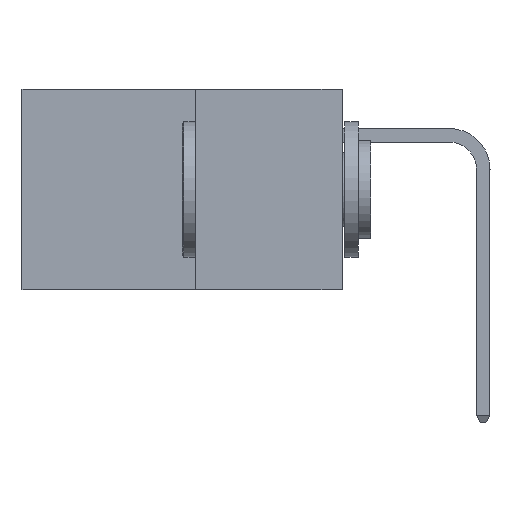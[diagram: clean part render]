
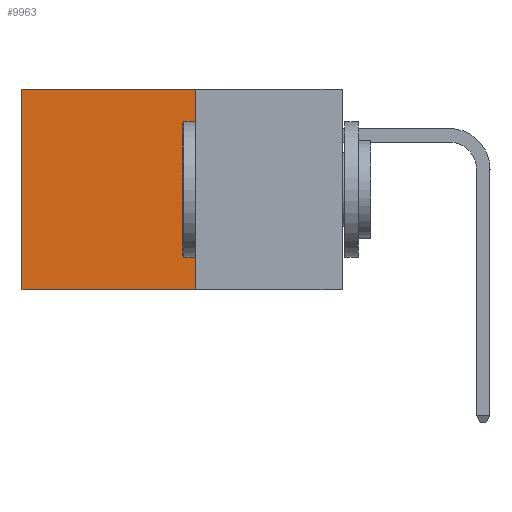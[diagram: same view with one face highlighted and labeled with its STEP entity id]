
A CAD part, left-side view. The second image highlights one B-rep face of the part: STEP entity #9963.
In plain terms, the highlighted planar face has unit normal (-1, 0, 0).
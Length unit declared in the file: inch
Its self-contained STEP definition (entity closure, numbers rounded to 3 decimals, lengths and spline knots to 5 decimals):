
#139 = DIRECTION ( 'NONE',  ( 0., 0., -1. ) ) ;
#162 = DIRECTION ( 'NONE',  ( 1., 0., 0. ) ) ;
#205 = CARTESIAN_POINT ( 'NONE',  ( 0.277, 0.27, -0.37 ) ) ;
#328 = CARTESIAN_POINT ( 'NONE',  ( 0.277, 0.27, -0.37 ) ) ;
#773 = PLANE ( 'NONE',  #18430 ) ;
#1620 = DIRECTION ( 'NONE',  ( 0., 1., 0. ) ) ;
#2046 = DIRECTION ( 'NONE',  ( 0., 0., -1. ) ) ;
#2365 = FACE_OUTER_BOUND ( 'NONE', #10256, .T. ) ;
#3644 = ORIENTED_EDGE ( 'NONE', *, *, #20527, .F. ) ;
#3859 = LINE ( 'NONE', #21439, #12169 ) ;
#5663 = EDGE_CURVE ( 'NONE', #18821, #10650, #12101, .T. ) ;
#6355 = DIRECTION ( 'NONE',  ( 0., 1., 0. ) ) ;
#7177 = VECTOR ( 'NONE', #15271, 39.37008 ) ;
#7465 = VERTEX_POINT ( 'NONE', #9952 ) ;
#9685 = VECTOR ( 'NONE', #2046, 39.37008 ) ;
#9881 = ORIENTED_EDGE ( 'NONE', *, *, #5663, .T. ) ;
#9952 = CARTESIAN_POINT ( 'NONE',  ( 0.277, 0.27, -0.37 ) ) ;
#9963 = ADVANCED_FACE ( 'NONE', ( #2365 ), #773, .F. ) ;
#10256 = EDGE_LOOP ( 'NONE', ( #9881, #3644, #15659, #20022 ) ) ;
#10650 = VERTEX_POINT ( 'NONE', #17677 ) ;
#11671 = EDGE_CURVE ( 'NONE', #20823, #7465, #14165, .T. ) ;
#11975 = VECTOR ( 'NONE', #6355, 39.37008 ) ;
#12101 = LINE ( 'NONE', #15163, #7177 ) ;
#12169 = VECTOR ( 'NONE', #1620, 39.37008 ) ;
#12953 = CARTESIAN_POINT ( 'NONE',  ( 0.277, 0.27, 0. ) ) ;
#14165 = LINE ( 'NONE', #328, #9685 ) ;
#15163 = CARTESIAN_POINT ( 'NONE',  ( 0.277, 0.59, -0.37 ) ) ;
#15271 = DIRECTION ( 'NONE',  ( 0., 0., -1. ) ) ;
#15561 = CARTESIAN_POINT ( 'NONE',  ( 0.277, 0.27, 0. ) ) ;
#15659 = ORIENTED_EDGE ( 'NONE', *, *, #11671, .F. ) ;
#16424 = LINE ( 'NONE', #12953, #11975 ) ;
#17677 = CARTESIAN_POINT ( 'NONE',  ( 0.277, 0.59, -0.37 ) ) ;
#18430 = AXIS2_PLACEMENT_3D ( 'NONE', #205, #162, #139 ) ;
#18821 = VERTEX_POINT ( 'NONE', #20507 ) ;
#19087 = EDGE_CURVE ( 'NONE', #20823, #18821, #16424, .T. ) ;
#20022 = ORIENTED_EDGE ( 'NONE', *, *, #19087, .T. ) ;
#20507 = CARTESIAN_POINT ( 'NONE',  ( 0.277, 0.59, 0. ) ) ;
#20527 = EDGE_CURVE ( 'NONE', #7465, #10650, #3859, .T. ) ;
#20823 = VERTEX_POINT ( 'NONE', #15561 ) ;
#21439 = CARTESIAN_POINT ( 'NONE',  ( 0.277, 0.27, -0.37 ) ) ;
